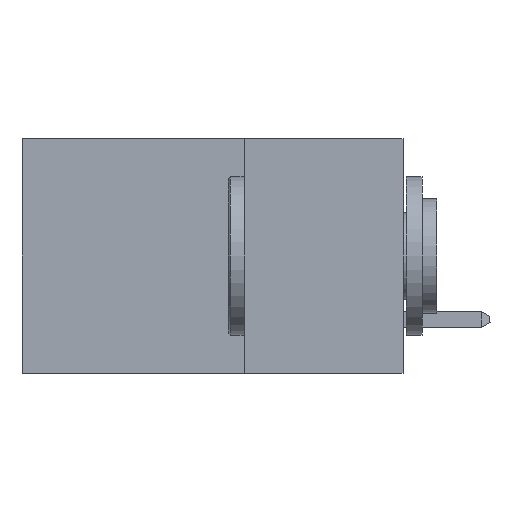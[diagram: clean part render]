
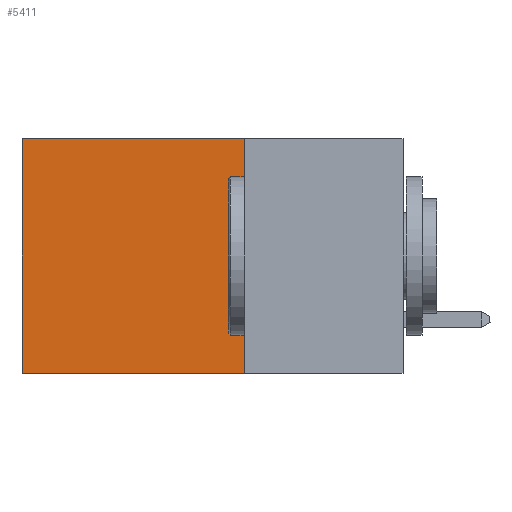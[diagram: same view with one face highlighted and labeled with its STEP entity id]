
A CAD part, left-side view. The second image highlights one B-rep face of the part: STEP entity #5411.
In plain terms, the highlighted planar face has unit normal (-1, 0, 0).
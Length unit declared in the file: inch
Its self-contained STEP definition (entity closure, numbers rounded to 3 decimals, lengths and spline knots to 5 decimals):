
#338 = PLANE ( 'NONE',  #28370 ) ;
#1994 = CARTESIAN_POINT ( 'NONE',  ( 0.2875, 0.6, 0. ) ) ;
#2016 = ORIENTED_EDGE ( 'NONE', *, *, #7273, .T. ) ;
#4108 = CARTESIAN_POINT ( 'NONE',  ( 0.2875, 0.25, 0. ) ) ;
#5411 = ADVANCED_FACE ( 'NONE', ( #8017 ), #338, .F. ) ;
#6390 = VERTEX_POINT ( 'NONE', #25660 ) ;
#7074 = CARTESIAN_POINT ( 'NONE',  ( 0.2875, 0.25, 0. ) ) ;
#7273 = EDGE_CURVE ( 'NONE', #6390, #20364, #25037, .T. ) ;
#7294 = DIRECTION ( 'NONE',  ( 0., 1., 0. ) ) ;
#7679 = ORIENTED_EDGE ( 'NONE', *, *, #26656, .T. ) ;
#7838 = CARTESIAN_POINT ( 'NONE',  ( 0.2875, 0.6, -0.37 ) ) ;
#8017 = FACE_OUTER_BOUND ( 'NONE', #16619, .T. ) ;
#9310 = EDGE_CURVE ( 'NONE', #28670, #15164, #30106, .T. ) ;
#10720 = VECTOR ( 'NONE', #21150, 39.37008 ) ;
#11503 = ORIENTED_EDGE ( 'NONE', *, *, #26970, .F. ) ;
#12259 = CARTESIAN_POINT ( 'NONE',  ( 0.2875, 0.6, 0. ) ) ;
#12365 = VECTOR ( 'NONE', #18003, 39.37008 ) ;
#14188 = DIRECTION ( 'NONE',  ( 1., 0., 0. ) ) ;
#14480 = DIRECTION ( 'NONE',  ( 0., 0., -1. ) ) ;
#15164 = VERTEX_POINT ( 'NONE', #7838 ) ;
#15165 = CARTESIAN_POINT ( 'NONE',  ( 0.2875, 0.25, -0.37 ) ) ;
#16619 = EDGE_LOOP ( 'NONE', ( #7679, #21222, #11503, #2016 ) ) ;
#17120 = LINE ( 'NONE', #12259, #25619 ) ;
#18003 = DIRECTION ( 'NONE',  ( 0., 0., -1. ) ) ;
#19685 = LINE ( 'NONE', #4108, #12365 ) ;
#20364 = VERTEX_POINT ( 'NONE', #1994 ) ;
#21150 = DIRECTION ( 'NONE',  ( 0., 1., 0. ) ) ;
#21222 = ORIENTED_EDGE ( 'NONE', *, *, #9310, .F. ) ;
#23761 = VECTOR ( 'NONE', #7294, 39.37008 ) ;
#24021 = DIRECTION ( 'NONE',  ( 0., 0., -1. ) ) ;
#25037 = LINE ( 'NONE', #7074, #10720 ) ;
#25619 = VECTOR ( 'NONE', #24021, 39.37008 ) ;
#25660 = CARTESIAN_POINT ( 'NONE',  ( 0.2875, 0.25, 0. ) ) ;
#26656 = EDGE_CURVE ( 'NONE', #20364, #15164, #17120, .T. ) ;
#26970 = EDGE_CURVE ( 'NONE', #6390, #28670, #19685, .T. ) ;
#28271 = CARTESIAN_POINT ( 'NONE',  ( 0.2875, 0.25, 0. ) ) ;
#28370 = AXIS2_PLACEMENT_3D ( 'NONE', #28271, #14188, #14480 ) ;
#28670 = VERTEX_POINT ( 'NONE', #15165 ) ;
#30106 = LINE ( 'NONE', #30407, #23761 ) ;
#30407 = CARTESIAN_POINT ( 'NONE',  ( 0.2875, 0.25, -0.37 ) ) ;
